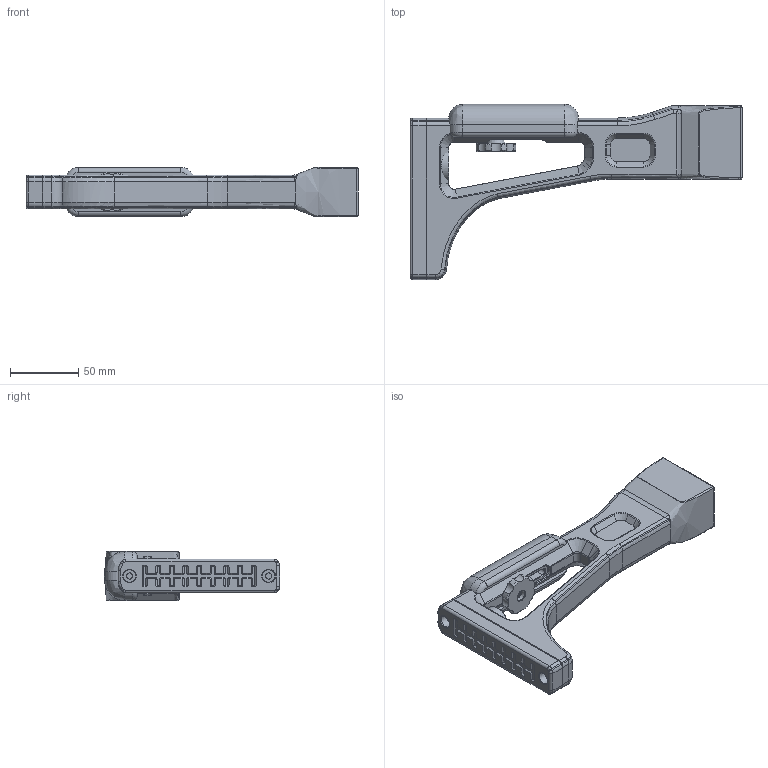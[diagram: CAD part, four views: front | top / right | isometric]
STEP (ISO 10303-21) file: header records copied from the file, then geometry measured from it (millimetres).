
FILE_DESCRIPTION(/* description */ (''),/* implementation_level */ '2;1');
FILE_NAME(/* name */ 'G36 stock.stp',/* time_stamp */ '2020-09-25T14:52:12+03:00',/* author */ (''),/* organization */ (''),/* preprocessor_version */ 'ST-DEVELOPER v15.2',/* originating_system */ 'Autodesk Translator Framework v2.0.0.5431',/* authorisation */ '');
FILE_SCHEMA (('AUTOMOTIVE_DESIGN { 1 0 10303 214 3 1 1 }'));
Length unit declared in the file: centimetre
Products named in the file (1): MOD9 G36 STOCK
Bounding box: 243.4 x 128.4 x 36 mm (x, y, z)
Volume: 331938.3 mm3; surface area: 69843.4 mm2
Topology: 4 solids, 4 shells, 573 faces, 1435 edges, 878 vertices
Faces by surface type: plane 183, bspline 166, cone 121, cylinder 76, torus 23, sphere 4
Full cylindrical faces by diameter (mm): 4.2 x1, 4.5 x4, 5 x1, 8 x1, 9 x2, 9.6 x1, 10 x1
Entity records: 24172 total; most frequent: CARTESIAN_POINT 11229, ORIENTED_EDGE 2808, DIRECTION 2526, EDGE_CURVE 1404, AXIS2_PLACEMENT_3D 912, VERTEX_POINT 874, LINE 702, VECTOR 702
